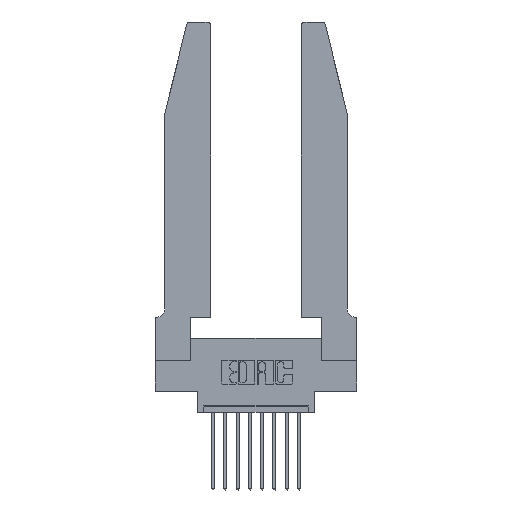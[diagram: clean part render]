
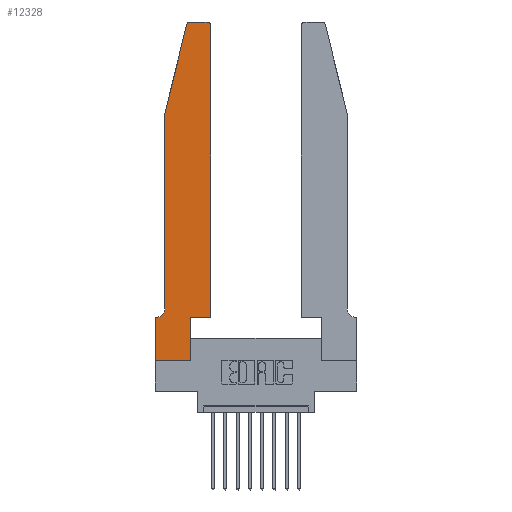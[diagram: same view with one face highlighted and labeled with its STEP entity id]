
A CAD part, top view. The second image highlights one B-rep face of the part: STEP entity #12328.
In plain terms, the highlighted planar face has unit normal (0, 0, 1).
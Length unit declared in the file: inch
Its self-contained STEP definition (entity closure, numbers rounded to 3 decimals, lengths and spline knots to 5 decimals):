
#329 = DIRECTION ( 'NONE',  ( 0., 1., 0. ) ) ;
#816 = ORIENTED_EDGE ( 'NONE', *, *, #11778, .T. ) ;
#845 = ORIENTED_EDGE ( 'NONE', *, *, #8842, .T. ) ;
#1216 = VERTEX_POINT ( 'NONE', #13119 ) ;
#1271 = LINE ( 'NONE', #8616, #2399 ) ;
#1365 = CARTESIAN_POINT ( 'NONE',  ( 0.0755, 0.35, 0.37 ) ) ;
#1800 = ORIENTED_EDGE ( 'NONE', *, *, #14427, .T. ) ;
#1901 = CARTESIAN_POINT ( 'NONE',  ( 0., 0., 0.37 ) ) ;
#1968 = LINE ( 'NONE', #4911, #8283 ) ;
#2002 = DIRECTION ( 'NONE',  ( 1., 0., 0. ) ) ;
#2150 = CARTESIAN_POINT ( 'NONE',  ( 0.0055, 0.42, 0.37 ) ) ;
#2399 = VECTOR ( 'NONE', #329, 39.37008 ) ;
#2469 = LINE ( 'NONE', #8564, #6736 ) ;
#2555 = CARTESIAN_POINT ( 'NONE',  ( 0., 0.35, 0.37 ) ) ;
#2670 = ORIENTED_EDGE ( 'NONE', *, *, #14495, .T. ) ;
#3075 = CIRCLE ( 'NONE', #6987, 0.03 ) ;
#3160 = DIRECTION ( 'NONE',  ( 0., 0., 1. ) ) ;
#3183 = PLANE ( 'NONE',  #5926 ) ;
#3480 = VECTOR ( 'NONE', #2002, 39.37008 ) ;
#3515 = DIRECTION ( 'NONE',  ( 1., 0., 0. ) ) ;
#3565 = DIRECTION ( 'NONE',  ( 0., -1., 0. ) ) ;
#3622 = VECTOR ( 'NONE', #5849, 39.37008 ) ;
#3660 = VERTEX_POINT ( 'NONE', #10201 ) ;
#3717 = CARTESIAN_POINT ( 'NONE',  ( 0.2605, 2.75, 0.37 ) ) ;
#4838 = LINE ( 'NONE', #13609, #8018 ) ;
#4911 = CARTESIAN_POINT ( 'NONE',  ( 0., 0., 0.37 ) ) ;
#5191 = EDGE_CURVE ( 'NONE', #8743, #9968, #3075, .T. ) ;
#5209 = CARTESIAN_POINT ( 'NONE',  ( 0.2865, 0.35, 0.37 ) ) ;
#5326 = CARTESIAN_POINT ( 'NONE',  ( 0.4205, 2.75, 0.37 ) ) ;
#5484 = DIRECTION ( 'NONE',  ( -1., 0., 0. ) ) ;
#5592 = CIRCLE ( 'NONE', #7034, 0.07 ) ;
#5632 = DIRECTION ( 'NONE',  ( 0., 0., -1. ) ) ;
#5849 = DIRECTION ( 'NONE',  ( -1., 0., 0. ) ) ;
#5926 = AXIS2_PLACEMENT_3D ( 'NONE', #2555, #15042, #3515 ) ;
#6162 = DIRECTION ( 'NONE',  ( -1., 0., 0. ) ) ;
#6432 = DIRECTION ( 'NONE',  ( 0., -1., 0. ) ) ;
#6434 = DIRECTION ( 'NONE',  ( 0., 1., 0. ) ) ;
#6718 = VERTEX_POINT ( 'NONE', #14036 ) ;
#6736 = VECTOR ( 'NONE', #13291, 39.37008 ) ;
#6854 = EDGE_LOOP ( 'NONE', ( #1800, #7156, #816, #13322, #8119, #15489, #13708, #845, #12168, #7424, #2670, #9728 ) ) ;
#6987 = AXIS2_PLACEMENT_3D ( 'NONE', #7744, #3160, #8946 ) ;
#7034 = AXIS2_PLACEMENT_3D ( 'NONE', #2150, #5632, #5484 ) ;
#7156 = ORIENTED_EDGE ( 'NONE', *, *, #10645, .T. ) ;
#7383 = DIRECTION ( 'NONE',  ( 1., 0., 0. ) ) ;
#7417 = LINE ( 'NONE', #3717, #7968 ) ;
#7424 = ORIENTED_EDGE ( 'NONE', *, *, #14815, .T. ) ;
#7492 = CIRCLE ( 'NONE', #10733, 0.03 ) ;
#7744 = CARTESIAN_POINT ( 'NONE',  ( 0.4205, 2.72, 0.37 ) ) ;
#7873 = VERTEX_POINT ( 'NONE', #14441 ) ;
#7968 = VECTOR ( 'NONE', #6162, 39.37008 ) ;
#8018 = VECTOR ( 'NONE', #6432, 39.37008 ) ;
#8119 = ORIENTED_EDGE ( 'NONE', *, *, #11083, .T. ) ;
#8207 = CARTESIAN_POINT ( 'NONE',  ( 0.0055, 0.35, 0.37 ) ) ;
#8283 = VECTOR ( 'NONE', #7383, 39.37008 ) ;
#8369 = CARTESIAN_POINT ( 'NONE',  ( 0., 0., 0.37 ) ) ;
#8389 = DIRECTION ( 'NONE',  ( 0., 0., 1. ) ) ;
#8564 = CARTESIAN_POINT ( 'NONE',  ( 0.0755, 2., 0.37 ) ) ;
#8616 = CARTESIAN_POINT ( 'NONE',  ( 0.4505, 0.35, 0.37 ) ) ;
#8742 = EDGE_CURVE ( 'NONE', #11118, #3660, #9788, .T. ) ;
#8743 = VERTEX_POINT ( 'NONE', #9469 ) ;
#8842 = EDGE_CURVE ( 'NONE', #14703, #9363, #1968, .T. ) ;
#8946 = DIRECTION ( 'NONE',  ( 1., 0., 0. ) ) ;
#9363 = VERTEX_POINT ( 'NONE', #14916 ) ;
#9469 = CARTESIAN_POINT ( 'NONE',  ( 0.4505, 2.72, 0.37 ) ) ;
#9496 = VECTOR ( 'NONE', #3565, 39.37008 ) ;
#9582 = DIRECTION ( 'NONE',  ( 1., 0., 0. ) ) ;
#9690 = CARTESIAN_POINT ( 'NONE',  ( 0.284, 2.72, 0.37 ) ) ;
#9728 = ORIENTED_EDGE ( 'NONE', *, *, #5191, .T. ) ;
#9763 = CARTESIAN_POINT ( 'NONE',  ( 0.25487, 2.72718, 0.37 ) ) ;
#9788 = LINE ( 'NONE', #1365, #3622 ) ;
#9968 = VERTEX_POINT ( 'NONE', #5326 ) ;
#10201 = CARTESIAN_POINT ( 'NONE',  ( 0., 0.35, 0.37 ) ) ;
#10207 = VERTEX_POINT ( 'NONE', #9763 ) ;
#10645 = EDGE_CURVE ( 'NONE', #10903, #10207, #7492, .T. ) ;
#10733 = AXIS2_PLACEMENT_3D ( 'NONE', #9690, #8389, #9582 ) ;
#10781 = LINE ( 'NONE', #11427, #3480 ) ;
#10903 = VERTEX_POINT ( 'NONE', #11348 ) ;
#11083 = EDGE_CURVE ( 'NONE', #6718, #11118, #5592, .T. ) ;
#11118 = VERTEX_POINT ( 'NONE', #8207 ) ;
#11348 = CARTESIAN_POINT ( 'NONE',  ( 0.284, 2.75, 0.37 ) ) ;
#11427 = CARTESIAN_POINT ( 'NONE',  ( 0.4505, 0.35, 0.37 ) ) ;
#11778 = EDGE_CURVE ( 'NONE', #10207, #7873, #2469, .T. ) ;
#11890 = EDGE_CURVE ( 'NONE', #7873, #6718, #4838, .T. ) ;
#12168 = ORIENTED_EDGE ( 'NONE', *, *, #14585, .T. ) ;
#12328 = ADVANCED_FACE ( 'NONE', ( #13134 ), #3183, .T. ) ;
#12430 = EDGE_CURVE ( 'NONE', #3660, #14703, #13519, .T. ) ;
#12798 = CARTESIAN_POINT ( 'NONE',  ( 0.4505, 0.35, 0.37 ) ) ;
#13119 = CARTESIAN_POINT ( 'NONE',  ( 0.2865, 0.35, 0.37 ) ) ;
#13134 = FACE_OUTER_BOUND ( 'NONE', #6854, .T. ) ;
#13291 = DIRECTION ( 'NONE',  ( -0.239, -0.971, 0. ) ) ;
#13322 = ORIENTED_EDGE ( 'NONE', *, *, #11890, .T. ) ;
#13519 = LINE ( 'NONE', #8369, #9496 ) ;
#13568 = VERTEX_POINT ( 'NONE', #12798 ) ;
#13609 = CARTESIAN_POINT ( 'NONE',  ( 0.0755, 2., 0.37 ) ) ;
#13708 = ORIENTED_EDGE ( 'NONE', *, *, #12430, .T. ) ;
#14036 = CARTESIAN_POINT ( 'NONE',  ( 0.0755, 0.42, 0.37 ) ) ;
#14409 = VECTOR ( 'NONE', #6434, 39.37008 ) ;
#14427 = EDGE_CURVE ( 'NONE', #9968, #10903, #7417, .T. ) ;
#14441 = CARTESIAN_POINT ( 'NONE',  ( 0.0755, 2., 0.37 ) ) ;
#14495 = EDGE_CURVE ( 'NONE', #13568, #8743, #1271, .T. ) ;
#14585 = EDGE_CURVE ( 'NONE', #9363, #1216, #15132, .T. ) ;
#14703 = VERTEX_POINT ( 'NONE', #1901 ) ;
#14815 = EDGE_CURVE ( 'NONE', #1216, #13568, #10781, .T. ) ;
#14916 = CARTESIAN_POINT ( 'NONE',  ( 0.2865, 0., 0.37 ) ) ;
#15042 = DIRECTION ( 'NONE',  ( 0., 0., 1. ) ) ;
#15132 = LINE ( 'NONE', #5209, #14409 ) ;
#15489 = ORIENTED_EDGE ( 'NONE', *, *, #8742, .T. ) ;
